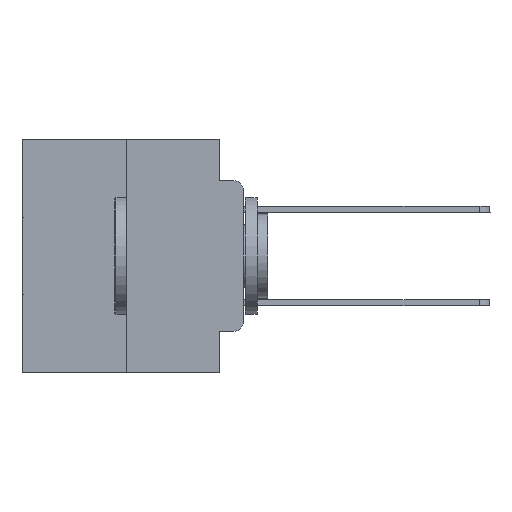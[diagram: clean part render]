
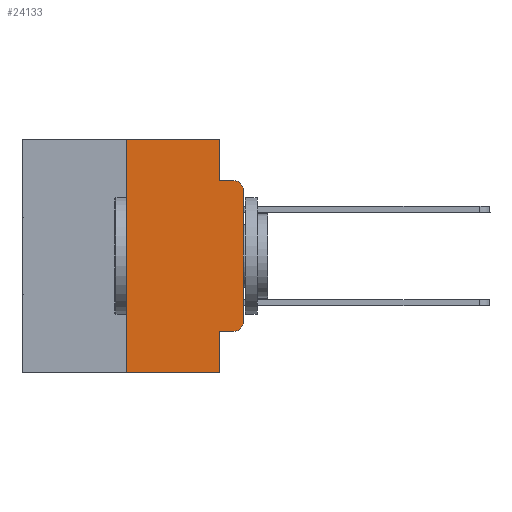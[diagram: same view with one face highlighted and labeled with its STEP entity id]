
A CAD part, left-side view. The second image highlights one B-rep face of the part: STEP entity #24133.
In plain terms, the highlighted planar face has unit normal (-1, 0, 0).
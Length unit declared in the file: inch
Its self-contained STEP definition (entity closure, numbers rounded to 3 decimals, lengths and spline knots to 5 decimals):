
#182 = CARTESIAN_POINT ( 'NONE',  ( 0., 0.25, 0. ) ) ;
#204 = VECTOR ( 'NONE', #24878, 39.37008 ) ;
#227 = AXIS2_PLACEMENT_3D ( 'NONE', #21960, #22119, #19263 ) ;
#1836 = LINE ( 'NONE', #11720, #17561 ) ;
#1930 = ORIENTED_EDGE ( 'NONE', *, *, #10297, .F. ) ;
#2487 = ORIENTED_EDGE ( 'NONE', *, *, #25065, .T. ) ;
#2636 = VERTEX_POINT ( 'NONE', #12131 ) ;
#2906 = CARTESIAN_POINT ( 'NONE',  ( 0., 0.051, -0.4115 ) ) ;
#3937 = AXIS2_PLACEMENT_3D ( 'NONE', #21182, #23404, #23717 ) ;
#4109 = ORIENTED_EDGE ( 'NONE', *, *, #13072, .T. ) ;
#4249 = ORIENTED_EDGE ( 'NONE', *, *, #26597, .T. ) ;
#4414 = ORIENTED_EDGE ( 'NONE', *, *, #8622, .F. ) ;
#5260 = DIRECTION ( 'NONE',  ( 0., 0., -1. ) ) ;
#5349 = DIRECTION ( 'NONE',  ( 0., 0., -1. ) ) ;
#5891 = CARTESIAN_POINT ( 'NONE',  ( 0., 0.051, 0. ) ) ;
#6215 = VERTEX_POINT ( 'NONE', #26120 ) ;
#7325 = VECTOR ( 'NONE', #19468, 39.37008 ) ;
#7452 = CARTESIAN_POINT ( 'NONE',  ( 0., 0.25, -0.5 ) ) ;
#8056 = DIRECTION ( 'NONE',  ( -1., 0., 0. ) ) ;
#8355 = CARTESIAN_POINT ( 'NONE',  ( 0., 0.051, -0.0885 ) ) ;
#8431 = VECTOR ( 'NONE', #19918, 39.37008 ) ;
#8622 = EDGE_CURVE ( 'NONE', #24646, #2636, #22482, .T. ) ;
#8748 = CARTESIAN_POINT ( 'NONE',  ( 0., 0., -0.3915 ) ) ;
#8901 = EDGE_LOOP ( 'NONE', ( #19740, #12419, #8988, #21954, #26475, #4414, #4109, #1930, #2487, #4249 ) ) ;
#8988 = ORIENTED_EDGE ( 'NONE', *, *, #30680, .F. ) ;
#9122 = CARTESIAN_POINT ( 'NONE',  ( 0., 0.02, -0.0885 ) ) ;
#9685 = DIRECTION ( 'NONE',  ( 0., -1., 0. ) ) ;
#10297 = EDGE_CURVE ( 'NONE', #16980, #26926, #1836, .T. ) ;
#10303 = VECTOR ( 'NONE', #24478, 39.37008 ) ;
#11414 = VECTOR ( 'NONE', #18281, 39.37008 ) ;
#11720 = CARTESIAN_POINT ( 'NONE',  ( 0., 0.051, 0. ) ) ;
#12071 = VECTOR ( 'NONE', #5260, 39.37008 ) ;
#12131 = CARTESIAN_POINT ( 'NONE',  ( 0., 0.25, 0. ) ) ;
#12133 = CIRCLE ( 'NONE', #29954, 0.02 ) ;
#12308 = VERTEX_POINT ( 'NONE', #20077 ) ;
#12419 = ORIENTED_EDGE ( 'NONE', *, *, #13783, .T. ) ;
#12687 = EDGE_CURVE ( 'NONE', #29458, #6215, #26876, .T. ) ;
#13072 = EDGE_CURVE ( 'NONE', #24646, #26926, #21468, .T. ) ;
#13613 = DIRECTION ( 'NONE',  ( 0., 0., -1. ) ) ;
#13783 = EDGE_CURVE ( 'NONE', #6215, #15816, #12133, .T. ) ;
#13858 = VERTEX_POINT ( 'NONE', #8355 ) ;
#14317 = FACE_OUTER_BOUND ( 'NONE', #8901, .T. ) ;
#15082 = CARTESIAN_POINT ( 'NONE',  ( 0., 0., 0. ) ) ;
#15621 = CARTESIAN_POINT ( 'NONE',  ( 0., 0.473, 0. ) ) ;
#15816 = VERTEX_POINT ( 'NONE', #9122 ) ;
#16980 = VERTEX_POINT ( 'NONE', #20588 ) ;
#17561 = VECTOR ( 'NONE', #13613, 39.37008 ) ;
#17671 = CIRCLE ( 'NONE', #3937, 0.02 ) ;
#17849 = LINE ( 'NONE', #15621, #204 ) ;
#18281 = DIRECTION ( 'NONE',  ( 0., -1., 0. ) ) ;
#19263 = DIRECTION ( 'NONE',  ( 0., 0., -1. ) ) ;
#19382 = VERTEX_POINT ( 'NONE', #26969 ) ;
#19468 = DIRECTION ( 'NONE',  ( 0., 0., 1. ) ) ;
#19740 = ORIENTED_EDGE ( 'NONE', *, *, #12687, .T. ) ;
#19918 = DIRECTION ( 'NONE',  ( 0., -1., 0. ) ) ;
#19973 = EDGE_CURVE ( 'NONE', #19382, #13858, #27710, .T. ) ;
#20077 = CARTESIAN_POINT ( 'NONE',  ( 0., 0.02, -0.4115 ) ) ;
#20588 = CARTESIAN_POINT ( 'NONE',  ( 0., 0.051, -0.4115 ) ) ;
#21182 = CARTESIAN_POINT ( 'NONE',  ( 0., 0.02, -0.3915 ) ) ;
#21468 = LINE ( 'NONE', #26740, #25963 ) ;
#21704 = LINE ( 'NONE', #2906, #8431 ) ;
#21954 = ORIENTED_EDGE ( 'NONE', *, *, #19973, .F. ) ;
#21960 = CARTESIAN_POINT ( 'NONE',  ( 0., 0.473, 0. ) ) ;
#22119 = DIRECTION ( 'NONE',  ( 1., 0., 0. ) ) ;
#22482 = LINE ( 'NONE', #182, #7325 ) ;
#23054 = CARTESIAN_POINT ( 'NONE',  ( 0., 0.051, -0.0885 ) ) ;
#23224 = LINE ( 'NONE', #23054, #11414 ) ;
#23404 = DIRECTION ( 'NONE',  ( -1., 0., 0. ) ) ;
#23717 = DIRECTION ( 'NONE',  ( 0., 0., -1. ) ) ;
#23858 = EDGE_CURVE ( 'NONE', #2636, #19382, #17849, .T. ) ;
#24133 = ADVANCED_FACE ( 'NONE', ( #14317 ), #28997, .F. ) ;
#24478 = DIRECTION ( 'NONE',  ( 0., 0., 1. ) ) ;
#24646 = VERTEX_POINT ( 'NONE', #7452 ) ;
#24878 = DIRECTION ( 'NONE',  ( 0., -1., 0. ) ) ;
#25065 = EDGE_CURVE ( 'NONE', #16980, #12308, #21704, .T. ) ;
#25963 = VECTOR ( 'NONE', #9685, 39.37008 ) ;
#26120 = CARTESIAN_POINT ( 'NONE',  ( 0., 0., -0.1085 ) ) ;
#26475 = ORIENTED_EDGE ( 'NONE', *, *, #23858, .F. ) ;
#26597 = EDGE_CURVE ( 'NONE', #12308, #29458, #17671, .T. ) ;
#26740 = CARTESIAN_POINT ( 'NONE',  ( 0., 0.473, -0.5 ) ) ;
#26876 = LINE ( 'NONE', #15082, #10303 ) ;
#26926 = VERTEX_POINT ( 'NONE', #27857 ) ;
#26969 = CARTESIAN_POINT ( 'NONE',  ( 0., 0.051, 0. ) ) ;
#27163 = CARTESIAN_POINT ( 'NONE',  ( 0., 0.02, -0.1085 ) ) ;
#27710 = LINE ( 'NONE', #5891, #12071 ) ;
#27857 = CARTESIAN_POINT ( 'NONE',  ( 0., 0.051, -0.5 ) ) ;
#28997 = PLANE ( 'NONE',  #227 ) ;
#29458 = VERTEX_POINT ( 'NONE', #8748 ) ;
#29954 = AXIS2_PLACEMENT_3D ( 'NONE', #27163, #8056, #5349 ) ;
#30680 = EDGE_CURVE ( 'NONE', #13858, #15816, #23224, .T. ) ;
